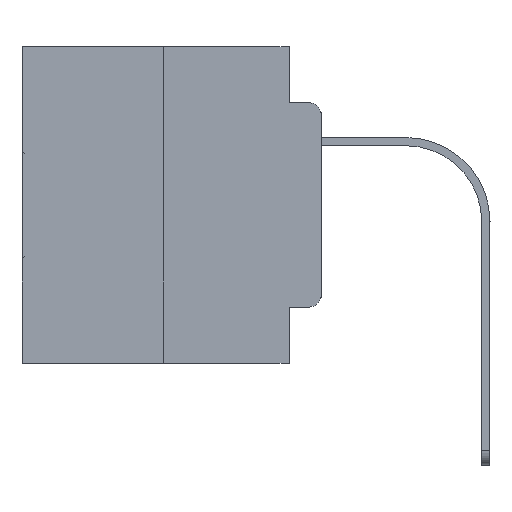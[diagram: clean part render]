
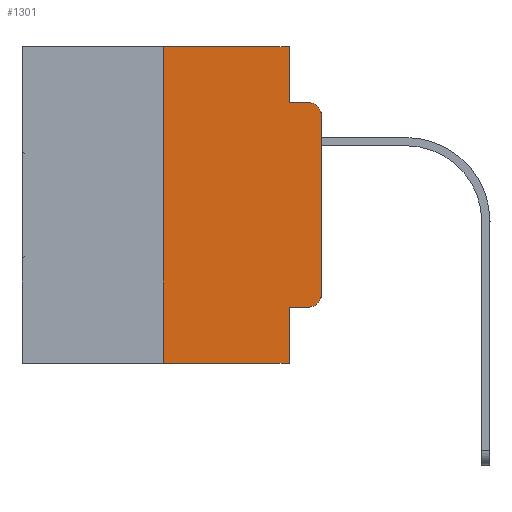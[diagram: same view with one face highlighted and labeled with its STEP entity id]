
A CAD part, left-side view. The second image highlights one B-rep face of the part: STEP entity #1301.
In plain terms, the highlighted planar face has unit normal (-1, 0, 0).
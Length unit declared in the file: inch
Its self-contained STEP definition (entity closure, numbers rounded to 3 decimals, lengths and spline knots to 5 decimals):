
#191 = PLANE ( 'NONE',  #12373 ) ;
#226 = EDGE_CURVE ( 'NONE', #7912, #14033, #20092, .T. ) ;
#366 = ORIENTED_EDGE ( 'NONE', *, *, #2763, .F. ) ;
#773 = CARTESIAN_POINT ( 'NONE',  ( 0., 0.051, -0.5 ) ) ;
#788 = DIRECTION ( 'NONE',  ( 0., 0., -1. ) ) ;
#821 = LINE ( 'NONE', #23388, #9631 ) ;
#931 = EDGE_CURVE ( 'NONE', #11285, #10776, #7597, .T. ) ;
#1301 = ADVANCED_FACE ( 'NONE', ( #4864 ), #191, .F. ) ;
#1389 = ORIENTED_EDGE ( 'NONE', *, *, #4630, .T. ) ;
#1956 = VECTOR ( 'NONE', #788, 39.37008 ) ;
#2100 = DIRECTION ( 'NONE',  ( 0., -1., 0. ) ) ;
#2243 = EDGE_CURVE ( 'NONE', #7912, #13925, #821, .T. ) ;
#2763 = EDGE_CURVE ( 'NONE', #11285, #13925, #3193, .T. ) ;
#3193 = LINE ( 'NONE', #26225, #1956 ) ;
#3649 = CARTESIAN_POINT ( 'NONE',  ( 0., 0., -0.1085 ) ) ;
#4626 = DIRECTION ( 'NONE',  ( -1., 0., 0. ) ) ;
#4630 = EDGE_CURVE ( 'NONE', #11170, #29138, #25587, .T. ) ;
#4864 = FACE_OUTER_BOUND ( 'NONE', #18493, .T. ) ;
#4905 = ORIENTED_EDGE ( 'NONE', *, *, #24044, .F. ) ;
#4927 = CARTESIAN_POINT ( 'NONE',  ( 0., 0.02, -0.3915 ) ) ;
#5180 = CARTESIAN_POINT ( 'NONE',  ( 0., 0.051, -0.4115 ) ) ;
#6127 = VERTEX_POINT ( 'NONE', #15441 ) ;
#6720 = CARTESIAN_POINT ( 'NONE',  ( 0., 0., 0. ) ) ;
#7417 = DIRECTION ( 'NONE',  ( 0., 0., -1. ) ) ;
#7496 = ORIENTED_EDGE ( 'NONE', *, *, #16487, .T. ) ;
#7597 = LINE ( 'NONE', #5180, #26487 ) ;
#7912 = VERTEX_POINT ( 'NONE', #19420 ) ;
#8005 = LINE ( 'NONE', #14673, #22259 ) ;
#9321 = VECTOR ( 'NONE', #25200, 39.37008 ) ;
#9572 = DIRECTION ( 'NONE',  ( 0., -1., 0. ) ) ;
#9591 = CARTESIAN_POINT ( 'NONE',  ( 0., 0., -0.3915 ) ) ;
#9631 = VECTOR ( 'NONE', #9572, 39.37008 ) ;
#9687 = CARTESIAN_POINT ( 'NONE',  ( 0., 0.02, -0.1085 ) ) ;
#9849 = EDGE_CURVE ( 'NONE', #17674, #29138, #22693, .T. ) ;
#10702 = CARTESIAN_POINT ( 'NONE',  ( 0., 0.051, -0.0885 ) ) ;
#10776 = VERTEX_POINT ( 'NONE', #17100 ) ;
#11170 = VERTEX_POINT ( 'NONE', #3649 ) ;
#11285 = VERTEX_POINT ( 'NONE', #25299 ) ;
#11980 = DIRECTION ( 'NONE',  ( 0., -1., 0. ) ) ;
#11998 = ORIENTED_EDGE ( 'NONE', *, *, #226, .F. ) ;
#12373 = AXIS2_PLACEMENT_3D ( 'NONE', #21058, #13776, #27741 ) ;
#12407 = VECTOR ( 'NONE', #17908, 39.37008 ) ;
#13057 = CARTESIAN_POINT ( 'NONE',  ( 0., 0.473, 0. ) ) ;
#13776 = DIRECTION ( 'NONE',  ( 1., 0., 0. ) ) ;
#13846 = DIRECTION ( 'NONE',  ( 0., 0., -1. ) ) ;
#13925 = VERTEX_POINT ( 'NONE', #773 ) ;
#14033 = VERTEX_POINT ( 'NONE', #26661 ) ;
#14613 = AXIS2_PLACEMENT_3D ( 'NONE', #4927, #4626, #13846 ) ;
#14673 = CARTESIAN_POINT ( 'NONE',  ( 0., 0.051, 0. ) ) ;
#15101 = CARTESIAN_POINT ( 'NONE',  ( 0., 0.02, -0.0885 ) ) ;
#15441 = CARTESIAN_POINT ( 'NONE',  ( 0., 0.051, 0. ) ) ;
#16487 = EDGE_CURVE ( 'NONE', #25120, #11170, #18209, .T. ) ;
#16804 = VECTOR ( 'NONE', #2100, 39.37008 ) ;
#17100 = CARTESIAN_POINT ( 'NONE',  ( 0., 0.02, -0.4115 ) ) ;
#17653 = CARTESIAN_POINT ( 'NONE',  ( 0., 0.25, 0. ) ) ;
#17674 = VERTEX_POINT ( 'NONE', #21611 ) ;
#17908 = DIRECTION ( 'NONE',  ( 0., -1., 0. ) ) ;
#18209 = LINE ( 'NONE', #6720, #9321 ) ;
#18493 = EDGE_LOOP ( 'NONE', ( #7496, #1389, #20282, #20907, #4905, #11998, #27178, #366, #21342, #24221 ) ) ;
#19097 = EDGE_CURVE ( 'NONE', #6127, #17674, #8005, .T. ) ;
#19420 = CARTESIAN_POINT ( 'NONE',  ( 0., 0.25, -0.5 ) ) ;
#19956 = CIRCLE ( 'NONE', #14613, 0.02 ) ;
#19962 = EDGE_CURVE ( 'NONE', #10776, #25120, #19956, .T. ) ;
#20092 = LINE ( 'NONE', #17653, #20147 ) ;
#20147 = VECTOR ( 'NONE', #24488, 39.37008 ) ;
#20266 = AXIS2_PLACEMENT_3D ( 'NONE', #9687, #28182, #7417 ) ;
#20282 = ORIENTED_EDGE ( 'NONE', *, *, #9849, .F. ) ;
#20907 = ORIENTED_EDGE ( 'NONE', *, *, #19097, .F. ) ;
#21058 = CARTESIAN_POINT ( 'NONE',  ( 0., 0.473, 0. ) ) ;
#21342 = ORIENTED_EDGE ( 'NONE', *, *, #931, .T. ) ;
#21611 = CARTESIAN_POINT ( 'NONE',  ( 0., 0.051, -0.0885 ) ) ;
#22259 = VECTOR ( 'NONE', #28771, 39.37008 ) ;
#22693 = LINE ( 'NONE', #10702, #16804 ) ;
#23388 = CARTESIAN_POINT ( 'NONE',  ( 0., 0.473, -0.5 ) ) ;
#24044 = EDGE_CURVE ( 'NONE', #14033, #6127, #29436, .T. ) ;
#24221 = ORIENTED_EDGE ( 'NONE', *, *, #19962, .T. ) ;
#24488 = DIRECTION ( 'NONE',  ( 0., 0., 1. ) ) ;
#25120 = VERTEX_POINT ( 'NONE', #9591 ) ;
#25200 = DIRECTION ( 'NONE',  ( 0., 0., 1. ) ) ;
#25299 = CARTESIAN_POINT ( 'NONE',  ( 0., 0.051, -0.4115 ) ) ;
#25587 = CIRCLE ( 'NONE', #20266, 0.02 ) ;
#26225 = CARTESIAN_POINT ( 'NONE',  ( 0., 0.051, 0. ) ) ;
#26487 = VECTOR ( 'NONE', #11980, 39.37008 ) ;
#26661 = CARTESIAN_POINT ( 'NONE',  ( 0., 0.25, 0. ) ) ;
#27178 = ORIENTED_EDGE ( 'NONE', *, *, #2243, .T. ) ;
#27741 = DIRECTION ( 'NONE',  ( 0., 0., -1. ) ) ;
#28182 = DIRECTION ( 'NONE',  ( -1., 0., 0. ) ) ;
#28771 = DIRECTION ( 'NONE',  ( 0., 0., -1. ) ) ;
#29138 = VERTEX_POINT ( 'NONE', #15101 ) ;
#29436 = LINE ( 'NONE', #13057, #12407 ) ;
